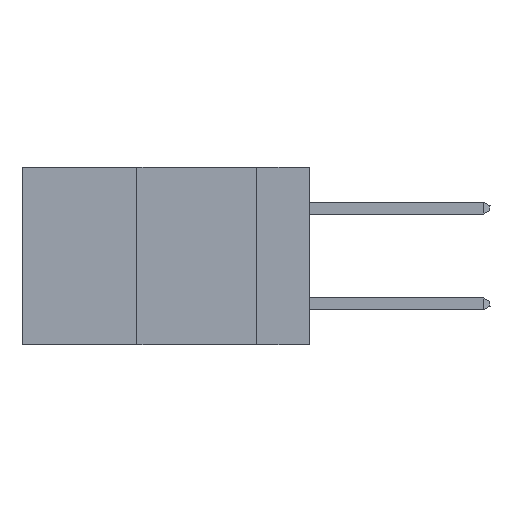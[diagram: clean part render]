
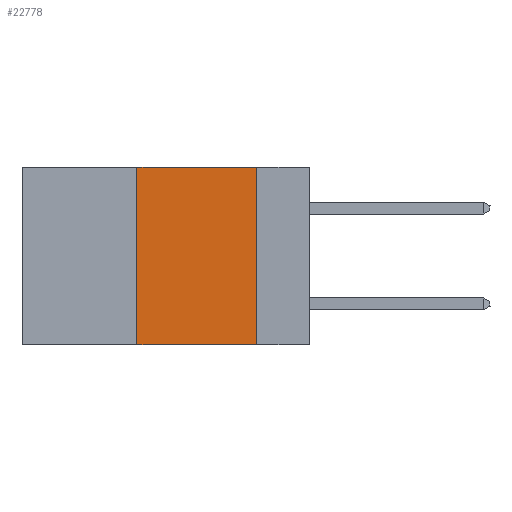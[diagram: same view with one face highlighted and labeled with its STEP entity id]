
A CAD part, left-side view. The second image highlights one B-rep face of the part: STEP entity #22778.
In plain terms, the highlighted planar face has unit normal (-1, 0, 0).
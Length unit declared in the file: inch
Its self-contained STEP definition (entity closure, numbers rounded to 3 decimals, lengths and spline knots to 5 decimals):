
#1378 = ORIENTED_EDGE ( 'NONE', *, *, #8631, .T. ) ;
#2149 = CARTESIAN_POINT ( 'NONE',  ( 0., 0.6, 0. ) ) ;
#3449 = ORIENTED_EDGE ( 'NONE', *, *, #13396, .F. ) ;
#3491 = LINE ( 'NONE', #23763, #22615 ) ;
#4301 = DIRECTION ( 'NONE',  ( 1., 0., 0. ) ) ;
#8631 = EDGE_CURVE ( 'NONE', #21415, #37082, #3491, .T. ) ;
#9931 = CARTESIAN_POINT ( 'NONE',  ( 0., 0.6, 0. ) ) ;
#9961 = VERTEX_POINT ( 'NONE', #21179 ) ;
#10408 = CARTESIAN_POINT ( 'NONE',  ( 0., 0.36, 0. ) ) ;
#10533 = DIRECTION ( 'NONE',  ( 0., 0., 1. ) ) ;
#10989 = VECTOR ( 'NONE', #10533, 39.37008 ) ;
#13396 = EDGE_CURVE ( 'NONE', #9961, #37082, #26950, .T. ) ;
#14957 = CARTESIAN_POINT ( 'NONE',  ( 0., 0.11, -0.37 ) ) ;
#16357 = EDGE_CURVE ( 'NONE', #24321, #9961, #27618, .T. ) ;
#16961 = CARTESIAN_POINT ( 'NONE',  ( 0., 0.36, 0. ) ) ;
#19008 = EDGE_LOOP ( 'NONE', ( #3449, #30584, #26140, #1378 ) ) ;
#20141 = VECTOR ( 'NONE', #24276, 39.37008 ) ;
#20580 = DIRECTION ( 'NONE',  ( 0., -1., 0. ) ) ;
#21179 = CARTESIAN_POINT ( 'NONE',  ( 0., 0.11, 0. ) ) ;
#21415 = VERTEX_POINT ( 'NONE', #29007 ) ;
#22313 = FACE_OUTER_BOUND ( 'NONE', #19008, .T. ) ;
#22615 = VECTOR ( 'NONE', #20580, 39.37008 ) ;
#22778 = ADVANCED_FACE ( 'NONE', ( #22313 ), #30383, .F. ) ;
#23763 = CARTESIAN_POINT ( 'NONE',  ( 0., 0.6, -0.37 ) ) ;
#24276 = DIRECTION ( 'NONE',  ( 0., 0., -1. ) ) ;
#24321 = VERTEX_POINT ( 'NONE', #16961 ) ;
#24537 = CARTESIAN_POINT ( 'NONE',  ( 0., 0.11, 0. ) ) ;
#25481 = EDGE_CURVE ( 'NONE', #21415, #24321, #35096, .T. ) ;
#26140 = ORIENTED_EDGE ( 'NONE', *, *, #25481, .F. ) ;
#26950 = LINE ( 'NONE', #24537, #20141 ) ;
#27618 = LINE ( 'NONE', #2149, #37202 ) ;
#29007 = CARTESIAN_POINT ( 'NONE',  ( 0., 0.36, -0.37 ) ) ;
#30383 = PLANE ( 'NONE',  #35866 ) ;
#30584 = ORIENTED_EDGE ( 'NONE', *, *, #16357, .F. ) ;
#33063 = DIRECTION ( 'NONE',  ( 0., 0., -1. ) ) ;
#35096 = LINE ( 'NONE', #10408, #10989 ) ;
#35866 = AXIS2_PLACEMENT_3D ( 'NONE', #9931, #4301, #33063 ) ;
#36598 = DIRECTION ( 'NONE',  ( 0., -1., 0. ) ) ;
#37082 = VERTEX_POINT ( 'NONE', #14957 ) ;
#37202 = VECTOR ( 'NONE', #36598, 39.37008 ) ;
